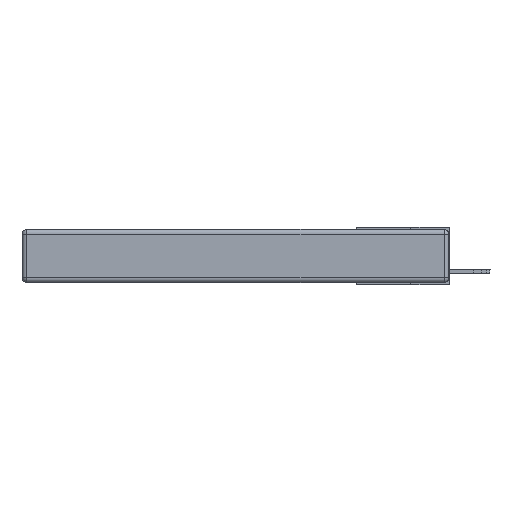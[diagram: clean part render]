
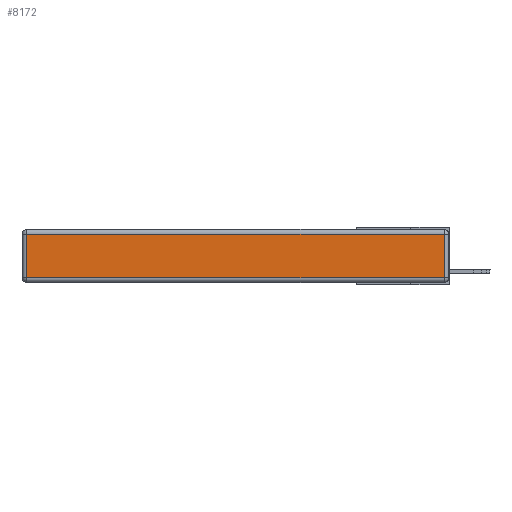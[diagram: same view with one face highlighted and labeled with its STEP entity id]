
A CAD part, left-side view. The second image highlights one B-rep face of the part: STEP entity #8172.
In plain terms, the highlighted planar face has unit normal (-1, 0, 0).
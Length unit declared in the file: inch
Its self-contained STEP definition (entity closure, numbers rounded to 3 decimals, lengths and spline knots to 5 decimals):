
#407 = ORIENTED_EDGE ( 'NONE', *, *, #7637, .T. ) ;
#705 = AXIS2_PLACEMENT_3D ( 'NONE', #2516, #15023, #1214 ) ;
#1214 = DIRECTION ( 'NONE',  ( 0., 0., 1. ) ) ;
#2160 = ORIENTED_EDGE ( 'NONE', *, *, #9021, .T. ) ;
#2516 = CARTESIAN_POINT ( 'NONE',  ( 0., 0., -0.343 ) ) ;
#3620 = LINE ( 'NONE', #15763, #13338 ) ;
#3717 = VERTEX_POINT ( 'NONE', #11196 ) ;
#3967 = VERTEX_POINT ( 'NONE', #8125 ) ;
#4526 = EDGE_LOOP ( 'NONE', ( #7803, #2160, #6118, #407 ) ) ;
#5749 = LINE ( 'NONE', #7060, #6615 ) ;
#6118 = ORIENTED_EDGE ( 'NONE', *, *, #11303, .T. ) ;
#6615 = VECTOR ( 'NONE', #16736, 39.37008 ) ;
#7060 = CARTESIAN_POINT ( 'NONE',  ( 0., 2.75, -0.03 ) ) ;
#7596 = LINE ( 'NONE', #14671, #16726 ) ;
#7637 = EDGE_CURVE ( 'NONE', #3967, #15645, #16010, .T. ) ;
#7703 = CARTESIAN_POINT ( 'NONE',  ( 0., 0.03, -0.03 ) ) ;
#7803 = ORIENTED_EDGE ( 'NONE', *, *, #12961, .T. ) ;
#8125 = CARTESIAN_POINT ( 'NONE',  ( 0., 2.72, -0.03 ) ) ;
#8172 = ADVANCED_FACE ( 'NONE', ( #14888 ), #10798, .T. ) ;
#9021 = EDGE_CURVE ( 'NONE', #3717, #11725, #3620, .T. ) ;
#10798 = PLANE ( 'NONE',  #705 ) ;
#11196 = CARTESIAN_POINT ( 'NONE',  ( 0., 0.03, -0.313 ) ) ;
#11303 = EDGE_CURVE ( 'NONE', #11725, #3967, #5749, .T. ) ;
#11342 = CARTESIAN_POINT ( 'NONE',  ( 0., 2.72, -0.313 ) ) ;
#11725 = VERTEX_POINT ( 'NONE', #7703 ) ;
#11821 = DIRECTION ( 'NONE',  ( 0., -1., 0. ) ) ;
#11867 = VECTOR ( 'NONE', #16533, 39.37008 ) ;
#12961 = EDGE_CURVE ( 'NONE', #15645, #3717, #7596, .T. ) ;
#13338 = VECTOR ( 'NONE', #17168, 39.37008 ) ;
#14671 = CARTESIAN_POINT ( 'NONE',  ( 0., 0., -0.313 ) ) ;
#14888 = FACE_OUTER_BOUND ( 'NONE', #4526, .T. ) ;
#15023 = DIRECTION ( 'NONE',  ( -1., 0., 0. ) ) ;
#15408 = CARTESIAN_POINT ( 'NONE',  ( 0., 2.72, -0.343 ) ) ;
#15645 = VERTEX_POINT ( 'NONE', #11342 ) ;
#15763 = CARTESIAN_POINT ( 'NONE',  ( 0., 0.03, -0.343 ) ) ;
#16010 = LINE ( 'NONE', #15408, #11867 ) ;
#16533 = DIRECTION ( 'NONE',  ( 0., 0., -1. ) ) ;
#16726 = VECTOR ( 'NONE', #11821, 39.37008 ) ;
#16736 = DIRECTION ( 'NONE',  ( 0., 1., 0. ) ) ;
#17168 = DIRECTION ( 'NONE',  ( 0., 0., 1. ) ) ;
